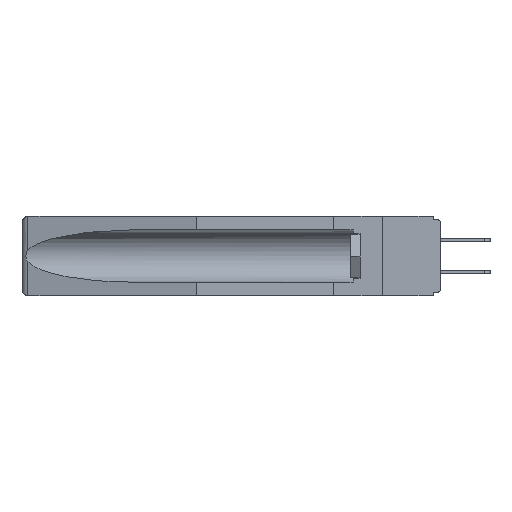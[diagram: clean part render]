
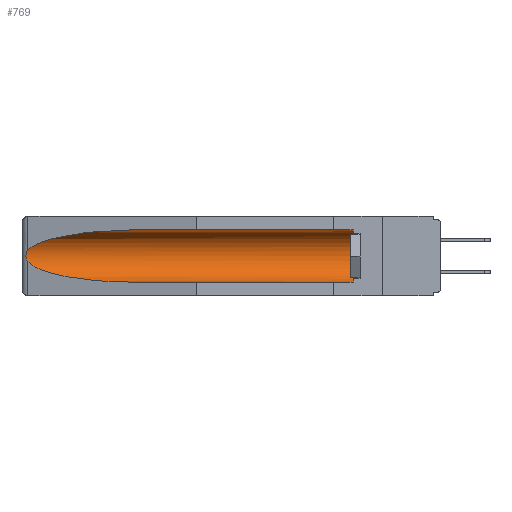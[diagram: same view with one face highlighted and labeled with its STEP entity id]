
A CAD part, left-side view. The second image highlights one B-rep face of the part: STEP entity #769.
In plain terms, the highlighted cylindrical face has radius 2.857 mm (diameter 5.715 mm), a partial arc.
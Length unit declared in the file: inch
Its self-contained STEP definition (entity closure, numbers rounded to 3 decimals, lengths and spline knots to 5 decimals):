
#119 = LINE ( 'NONE', #6989, #12764 ) ;
#135 = CARTESIAN_POINT ( 'NONE',  ( 0.26537, 1.52718, -0.19328 ) ) ;
#491 = VERTEX_POINT ( 'NONE', #13167 ) ;
#769 = ADVANCED_FACE ( 'NONE', ( #14352 ), #2399, .F. ) ;
#899 = CARTESIAN_POINT ( 'NONE',  ( 0.26654, 1.53092, -0.15636 ) ) ;
#952 = ORIENTED_EDGE ( 'NONE', *, *, #10415, .F. ) ;
#1095 = CARTESIAN_POINT ( 'NONE',  ( 0.2675, 1.53308, -0.16763 ) ) ;
#1672 = ORIENTED_EDGE ( 'NONE', *, *, #17708, .T. ) ;
#2004 = VERTEX_POINT ( 'NONE', #11870 ) ;
#2268 = VERTEX_POINT ( 'NONE', #10238 ) ;
#2353 = CARTESIAN_POINT ( 'NONE',  ( 0.2673, 1.53269, -0.17917 ) ) ;
#2399 = CYLINDRICAL_SURFACE ( 'NONE', #6276, 0.1125 ) ;
#2431 = CARTESIAN_POINT ( 'NONE',  ( 0.26597, 1.52961, -0.15275 ) ) ;
#2620 = CARTESIAN_POINT ( 'NONE',  ( 0.26537, 1.52718, -0.14972 ) ) ;
#3382 = CARTESIAN_POINT ( 'NONE',  ( 0.21114, 1.30732, -0.284 ) ) ;
#3391 = CARTESIAN_POINT ( 'NONE',  ( 0.155, 1.07973, -0.059 ) ) ;
#3410 =( BOUNDED_CURVE ( )  B_SPLINE_CURVE ( 3, ( #18546, #17272, #17153, #12797 ),
 .UNSPECIFIED., .F., .F. ) 
 B_SPLINE_CURVE_WITH_KNOTS ( ( 4, 4 ),
 ( 4.71239, 6.08839 ),
 .UNSPECIFIED. ) 
 CURVE ( )  GEOMETRIC_REPRESENTATION_ITEM ( )  RATIONAL_B_SPLINE_CURVE ( ( 1., 0.848, 0.848, 1. ) ) 
 REPRESENTATION_ITEM ( '' )  );
#4099 = DIRECTION ( 'NONE',  ( 0., -1., 0. ) ) ;
#4250 = CARTESIAN_POINT ( 'NONE',  ( 0.155, 0.126, -0.284 ) ) ;
#4823 =( BOUNDED_CURVE ( )  B_SPLINE_CURVE ( 3, ( #15199, #9241, #3382, #9365 ),
 .UNSPECIFIED., .F., .F. ) 
 B_SPLINE_CURVE_WITH_KNOTS ( ( 4, 4 ),
 ( 0.1948, 1.5708 ),
 .UNSPECIFIED. ) 
 CURVE ( )  GEOMETRIC_REPRESENTATION_ITEM ( )  RATIONAL_B_SPLINE_CURVE ( ( 1., 0.848, 0.848, 1. ) ) 
 REPRESENTATION_ITEM ( '' )  );
#5218 = VERTEX_POINT ( 'NONE', #4250 ) ;
#5471 = CARTESIAN_POINT ( 'NONE',  ( 0.155, -0.30754, -0.284 ) ) ;
#5920 = ORIENTED_EDGE ( 'NONE', *, *, #8145, .T. ) ;
#6276 = AXIS2_PLACEMENT_3D ( 'NONE', #18333, #14303, #11268 ) ;
#6830 = EDGE_CURVE ( 'NONE', #8936, #491, #4823, .T. ) ;
#6853 = DIRECTION ( 'NONE',  ( 0., 1., 0. ) ) ;
#6989 = CARTESIAN_POINT ( 'NONE',  ( 0.155, -0.30754, -0.059 ) ) ;
#7428 = B_SPLINE_CURVE_WITH_KNOTS ( 'NONE', 3,
 ( #2620, #2431, #899, #12715, #1095, #18465, #2353, #9925, #11221, #12843 ),
 .UNSPECIFIED., .F., .F.,
 ( 4, 2, 2, 2, 4 ),
 ( 0., 0.00029, 0.00058, 0.00087, 0.00117 ),
 .UNSPECIFIED. ) ;
#8145 = EDGE_CURVE ( 'NONE', #17383, #2004, #3410, .T. ) ;
#8689 = DIRECTION ( 'NONE',  ( 0., 0., 1. ) ) ;
#8936 = VERTEX_POINT ( 'NONE', #135 ) ;
#9241 = CARTESIAN_POINT ( 'NONE',  ( 0.25451, 1.48313, -0.24835 ) ) ;
#9365 = CARTESIAN_POINT ( 'NONE',  ( 0.155, 1.07973, -0.284 ) ) ;
#9712 = DIRECTION ( 'NONE',  ( 0., 1., 0. ) ) ;
#9925 = CARTESIAN_POINT ( 'NONE',  ( 0.26655, 1.53094, -0.18657 ) ) ;
#10238 = CARTESIAN_POINT ( 'NONE',  ( 0.155, 0.126, -0.059 ) ) ;
#10415 = EDGE_CURVE ( 'NONE', #5218, #491, #10975, .T. ) ;
#10673 = EDGE_CURVE ( 'NONE', #5218, #2268, #13731, .T. ) ;
#10829 = ORIENTED_EDGE ( 'NONE', *, *, #15065, .T. ) ;
#10975 = LINE ( 'NONE', #5471, #17877 ) ;
#11123 = CARTESIAN_POINT ( 'NONE',  ( 0.155, 0.126, -0.1715 ) ) ;
#11221 = CARTESIAN_POINT ( 'NONE',  ( 0.26597, 1.5296, -0.19026 ) ) ;
#11268 = DIRECTION ( 'NONE',  ( 0., 0., 1. ) ) ;
#11355 = ORIENTED_EDGE ( 'NONE', *, *, #6830, .T. ) ;
#11870 = CARTESIAN_POINT ( 'NONE',  ( 0.26537, 1.52718, -0.14972 ) ) ;
#12398 = ORIENTED_EDGE ( 'NONE', *, *, #10673, .T. ) ;
#12715 = CARTESIAN_POINT ( 'NONE',  ( 0.2673, 1.5327, -0.16383 ) ) ;
#12764 = VECTOR ( 'NONE', #6853, 39.37008 ) ;
#12797 = CARTESIAN_POINT ( 'NONE',  ( 0.26537, 1.52718, -0.14972 ) ) ;
#12843 = CARTESIAN_POINT ( 'NONE',  ( 0.26537, 1.52718, -0.19328 ) ) ;
#13167 = CARTESIAN_POINT ( 'NONE',  ( 0.155, 1.07973, -0.284 ) ) ;
#13731 = CIRCLE ( 'NONE', #18932, 0.1125 ) ;
#14303 = DIRECTION ( 'NONE',  ( 0., 1., 0. ) ) ;
#14352 = FACE_OUTER_BOUND ( 'NONE', #15427, .T. ) ;
#15065 = EDGE_CURVE ( 'NONE', #2004, #8936, #7428, .T. ) ;
#15199 = CARTESIAN_POINT ( 'NONE',  ( 0.26537, 1.52718, -0.19328 ) ) ;
#15427 = EDGE_LOOP ( 'NONE', ( #5920, #10829, #11355, #952, #12398, #1672 ) ) ;
#17153 = CARTESIAN_POINT ( 'NONE',  ( 0.25451, 1.48313, -0.09465 ) ) ;
#17272 = CARTESIAN_POINT ( 'NONE',  ( 0.21114, 1.30732, -0.059 ) ) ;
#17383 = VERTEX_POINT ( 'NONE', #3391 ) ;
#17708 = EDGE_CURVE ( 'NONE', #2268, #17383, #119, .T. ) ;
#17877 = VECTOR ( 'NONE', #9712, 39.37008 ) ;
#18333 = CARTESIAN_POINT ( 'NONE',  ( 0.155, -0.30754, -0.1715 ) ) ;
#18465 = CARTESIAN_POINT ( 'NONE',  ( 0.2675, 1.53308, -0.17534 ) ) ;
#18546 = CARTESIAN_POINT ( 'NONE',  ( 0.155, 1.07973, -0.059 ) ) ;
#18932 = AXIS2_PLACEMENT_3D ( 'NONE', #11123, #4099, #8689 ) ;
